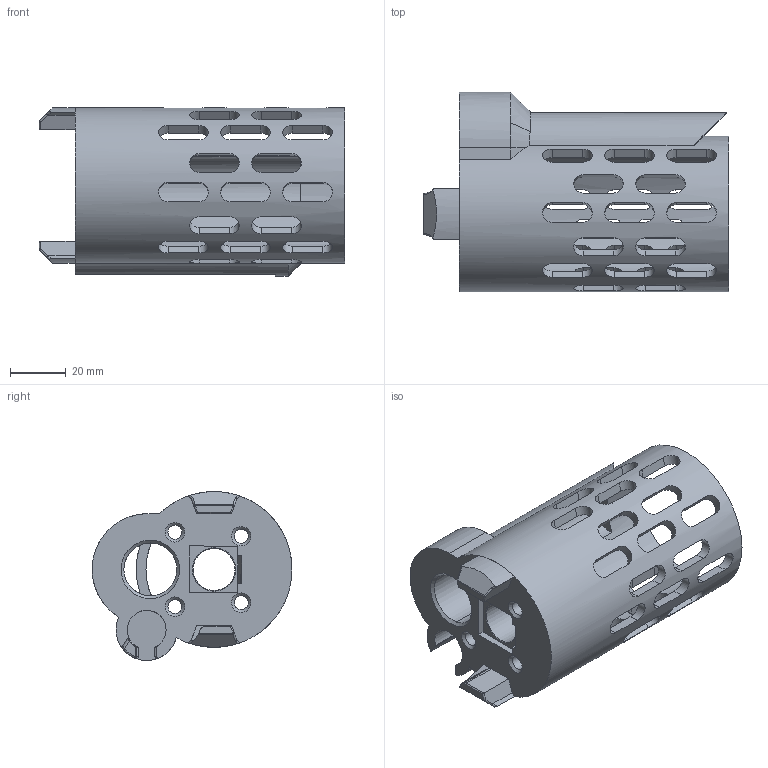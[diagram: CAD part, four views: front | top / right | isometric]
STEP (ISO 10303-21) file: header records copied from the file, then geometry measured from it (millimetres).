
FILE_DESCRIPTION(/* description */ ('STEP AP214'),/* implementation_level */ '2;1');
FILE_NAME(/* author */ (''),/* organization */ (''),/* preprocessor_version */ 'ST-DEVELOPER v18.1',/* originating_system */ ' ',/* authorisation */ ' ');
FILE_SCHEMA (('AUTOMOTIVE_DESIGN {1 0 10303 214 3 1 1}'));
Length unit declared in the file: metre
Products named in the file (1): MOD9_GOAT_TEC_barrel_retainer v8
Bounding box: 110.02 x 71.88 x 60.72 mm (x, y, z)
Volume: 104750.7 mm3; surface area: 43293.6 mm2
Topology: 1 solids, 1 shells, 240 faces, 676 edges, 438 vertices
Faces by surface type: cylinder 109, plane 104, cone 9, bspline 8, torus 5, sphere 5
Full cylindrical faces by diameter (mm): 5 x4, 15.1 x1, 49 x1, 56 x1
Entity records: 8481 total; most frequent: CARTESIAN_POINT 2460, ORIENTED_EDGE 1310, DIRECTION 1076, EDGE_CURVE 655, VERTEX_POINT 433, LINE 376, VECTOR 376, AXIS2_PLACEMENT_3D 350
